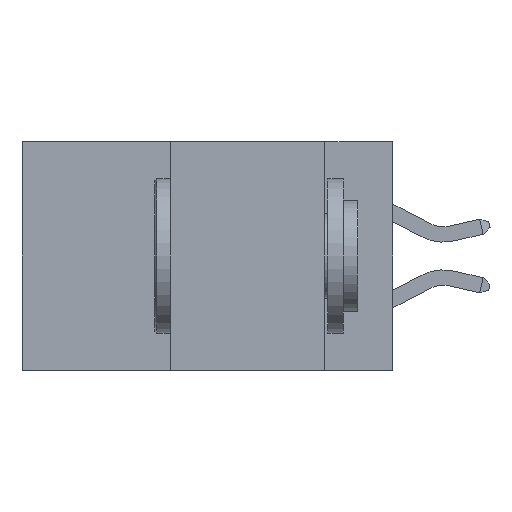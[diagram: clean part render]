
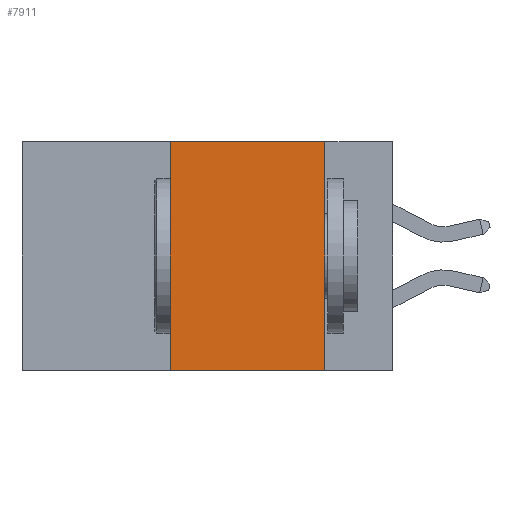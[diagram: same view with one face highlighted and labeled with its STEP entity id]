
A CAD part, left-side view. The second image highlights one B-rep face of the part: STEP entity #7911.
In plain terms, the highlighted planar face has unit normal (-1, 0, 0).
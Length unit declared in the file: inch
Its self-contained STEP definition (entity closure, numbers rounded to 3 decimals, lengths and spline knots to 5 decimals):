
#774 = ORIENTED_EDGE ( 'NONE', *, *, #7549, .F. ) ;
#814 = ORIENTED_EDGE ( 'NONE', *, *, #14396, .F. ) ;
#1028 = ORIENTED_EDGE ( 'NONE', *, *, #6639, .F. ) ;
#1082 = ORIENTED_EDGE ( 'NONE', *, *, #3016, .T. ) ;
#1521 = LINE ( 'NONE', #3402, #11307 ) ;
#2004 = PLANE ( 'NONE',  #13262 ) ;
#2412 = VERTEX_POINT ( 'NONE', #7482 ) ;
#3016 = EDGE_CURVE ( 'NONE', #5210, #2412, #6127, .T. ) ;
#3402 = CARTESIAN_POINT ( 'NONE',  ( 0., 0.6, 0. ) ) ;
#3470 = DIRECTION ( 'NONE',  ( 0., 0., -1. ) ) ;
#3900 = LINE ( 'NONE', #5957, #16636 ) ;
#4087 = VERTEX_POINT ( 'NONE', #15762 ) ;
#4156 = CARTESIAN_POINT ( 'NONE',  ( 0., 0.36, -0.37 ) ) ;
#5210 = VERTEX_POINT ( 'NONE', #4156 ) ;
#5400 = CARTESIAN_POINT ( 'NONE',  ( 0., 0.36, 0. ) ) ;
#5785 = VECTOR ( 'NONE', #10549, 39.37008 ) ;
#5957 = CARTESIAN_POINT ( 'NONE',  ( 0., 0.36, 0. ) ) ;
#6127 = LINE ( 'NONE', #10047, #12470 ) ;
#6639 = EDGE_CURVE ( 'NONE', #5210, #12623, #3900, .T. ) ;
#7226 = DIRECTION ( 'NONE',  ( 0., 0., 1. ) ) ;
#7482 = CARTESIAN_POINT ( 'NONE',  ( 0., 0.11, -0.37 ) ) ;
#7549 = EDGE_CURVE ( 'NONE', #4087, #2412, #9286, .T. ) ;
#7911 = ADVANCED_FACE ( 'NONE', ( #16594 ), #2004, .F. ) ;
#9286 = LINE ( 'NONE', #12972, #5785 ) ;
#10031 = DIRECTION ( 'NONE',  ( 0., -1., 0. ) ) ;
#10047 = CARTESIAN_POINT ( 'NONE',  ( 0., 0.6, -0.37 ) ) ;
#10549 = DIRECTION ( 'NONE',  ( 0., 0., -1. ) ) ;
#11064 = EDGE_LOOP ( 'NONE', ( #774, #814, #1028, #1082 ) ) ;
#11252 = DIRECTION ( 'NONE',  ( 1., 0., 0. ) ) ;
#11307 = VECTOR ( 'NONE', #13728, 39.37008 ) ;
#12470 = VECTOR ( 'NONE', #10031, 39.37008 ) ;
#12623 = VERTEX_POINT ( 'NONE', #5400 ) ;
#12972 = CARTESIAN_POINT ( 'NONE',  ( 0., 0.11, 0. ) ) ;
#13262 = AXIS2_PLACEMENT_3D ( 'NONE', #16222, #11252, #3470 ) ;
#13728 = DIRECTION ( 'NONE',  ( 0., -1., 0. ) ) ;
#14396 = EDGE_CURVE ( 'NONE', #12623, #4087, #1521, .T. ) ;
#15762 = CARTESIAN_POINT ( 'NONE',  ( 0., 0.11, 0. ) ) ;
#16222 = CARTESIAN_POINT ( 'NONE',  ( 0., 0.6, 0. ) ) ;
#16594 = FACE_OUTER_BOUND ( 'NONE', #11064, .T. ) ;
#16636 = VECTOR ( 'NONE', #7226, 39.37008 ) ;
